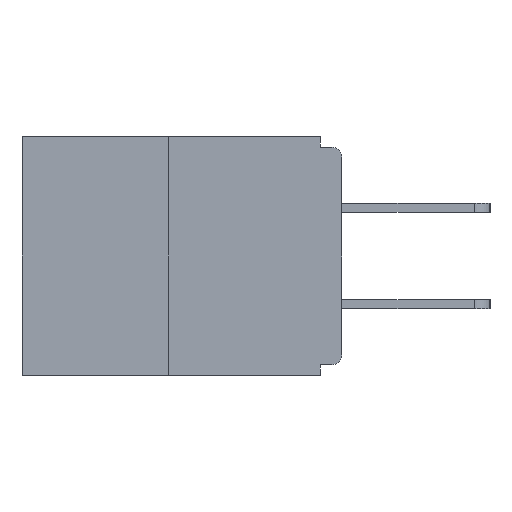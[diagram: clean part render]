
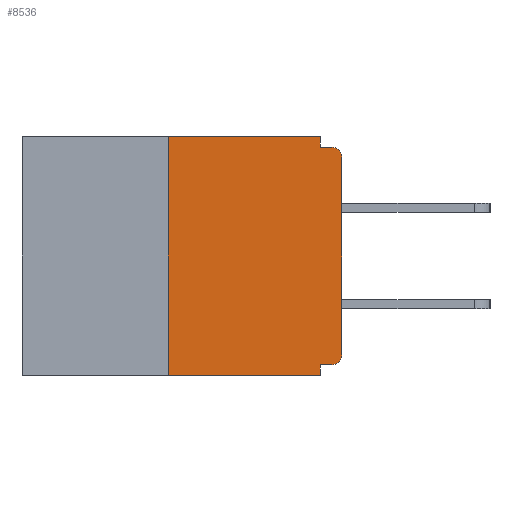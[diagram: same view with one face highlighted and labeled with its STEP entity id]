
A CAD part, left-side view. The second image highlights one B-rep face of the part: STEP entity #8536.
In plain terms, the highlighted planar face has unit normal (-1, 0, 0).
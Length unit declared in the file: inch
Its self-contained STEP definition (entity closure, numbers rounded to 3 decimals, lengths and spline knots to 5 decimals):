
#121 = DIRECTION ( 'NONE',  ( -1., 0., 0. ) ) ;
#288 = DIRECTION ( 'NONE',  ( 0., -1., 0. ) ) ;
#297 = VERTEX_POINT ( 'NONE', #10565 ) ;
#346 = FACE_OUTER_BOUND ( 'NONE', #8840, .T. ) ;
#440 = LINE ( 'NONE', #13650, #11971 ) ;
#607 = DIRECTION ( 'NONE',  ( 0., 0., 1. ) ) ;
#777 = CARTESIAN_POINT ( 'NONE',  ( 0., 0.015, -0.313 ) ) ;
#892 = AXIS2_PLACEMENT_3D ( 'NONE', #9704, #121, #13093 ) ;
#996 = ORIENTED_EDGE ( 'NONE', *, *, #9010, .F. ) ;
#1047 = VERTEX_POINT ( 'NONE', #8521 ) ;
#1098 = CARTESIAN_POINT ( 'NONE',  ( 0., 0.015, -0.328 ) ) ;
#1239 = ORIENTED_EDGE ( 'NONE', *, *, #13432, .F. ) ;
#1295 = ORIENTED_EDGE ( 'NONE', *, *, #5062, .F. ) ;
#1489 = PLANE ( 'NONE',  #9682 ) ;
#1593 = VERTEX_POINT ( 'NONE', #3477 ) ;
#2146 = CARTESIAN_POINT ( 'NONE',  ( 0., 0.25, 0. ) ) ;
#2199 = CARTESIAN_POINT ( 'NONE',  ( 0., 0., -0.03 ) ) ;
#2522 = DIRECTION ( 'NONE',  ( 0., -1., 0. ) ) ;
#2578 = CARTESIAN_POINT ( 'NONE',  ( 0., 0.46, 0. ) ) ;
#2584 = ORIENTED_EDGE ( 'NONE', *, *, #3520, .T. ) ;
#2741 = DIRECTION ( 'NONE',  ( 0., 0., -1. ) ) ;
#3351 = VERTEX_POINT ( 'NONE', #14067 ) ;
#3357 = VERTEX_POINT ( 'NONE', #12933 ) ;
#3477 = CARTESIAN_POINT ( 'NONE',  ( 0., 0.031, -0.343 ) ) ;
#3520 = EDGE_CURVE ( 'NONE', #12485, #3357, #7251, .T. ) ;
#3584 = CARTESIAN_POINT ( 'NONE',  ( 0., 0.46, 0. ) ) ;
#3701 = ORIENTED_EDGE ( 'NONE', *, *, #10935, .F. ) ;
#3854 = DIRECTION ( 'NONE',  ( 0., -1., 0. ) ) ;
#3901 = LINE ( 'NONE', #6438, #13106 ) ;
#4170 = EDGE_CURVE ( 'NONE', #7178, #3351, #13710, .T. ) ;
#4305 = CARTESIAN_POINT ( 'NONE',  ( 0., 0.25, 0. ) ) ;
#4355 = ORIENTED_EDGE ( 'NONE', *, *, #8280, .T. ) ;
#5062 = EDGE_CURVE ( 'NONE', #297, #10849, #440, .T. ) ;
#5086 = DIRECTION ( 'NONE',  ( 0., 0., -1. ) ) ;
#5302 = CARTESIAN_POINT ( 'NONE',  ( 0., 0.031, -0.343 ) ) ;
#5489 = ORIENTED_EDGE ( 'NONE', *, *, #10494, .F. ) ;
#5531 = VECTOR ( 'NONE', #607, 39.37008 ) ;
#5757 = LINE ( 'NONE', #8891, #9996 ) ;
#5879 = CARTESIAN_POINT ( 'NONE',  ( 0., 0.031, -0.328 ) ) ;
#6438 = CARTESIAN_POINT ( 'NONE',  ( 0., 0., 0. ) ) ;
#6779 = VECTOR ( 'NONE', #3854, 39.37008 ) ;
#6799 = DIRECTION ( 'NONE',  ( 0., 1., 0. ) ) ;
#6903 = LINE ( 'NONE', #2146, #5531 ) ;
#7178 = VERTEX_POINT ( 'NONE', #2199 ) ;
#7251 = CIRCLE ( 'NONE', #10456, 0.015 ) ;
#7663 = VECTOR ( 'NONE', #2522, 39.37008 ) ;
#7943 = LINE ( 'NONE', #3584, #13074 ) ;
#8221 = ORIENTED_EDGE ( 'NONE', *, *, #8474, .F. ) ;
#8280 = EDGE_CURVE ( 'NONE', #1047, #1593, #13930, .T. ) ;
#8474 = EDGE_CURVE ( 'NONE', #12485, #11956, #5757, .T. ) ;
#8519 = CARTESIAN_POINT ( 'NONE',  ( 0., 0.031, -0.015 ) ) ;
#8521 = CARTESIAN_POINT ( 'NONE',  ( 0., 0.25, -0.343 ) ) ;
#8536 = ADVANCED_FACE ( 'NONE', ( #346 ), #1489, .F. ) ;
#8538 = DIRECTION ( 'NONE',  ( 0., 0., 1. ) ) ;
#8840 = EDGE_LOOP ( 'NONE', ( #996, #1239, #4355, #3701, #8221, #2584, #9899, #11699, #5489, #1295 ) ) ;
#8869 = LINE ( 'NONE', #10265, #7663 ) ;
#8891 = CARTESIAN_POINT ( 'NONE',  ( 0., 0., -0.328 ) ) ;
#9010 = EDGE_CURVE ( 'NONE', #11221, #297, #7943, .T. ) ;
#9227 = DIRECTION ( 'NONE',  ( 1., 0., 0. ) ) ;
#9370 = CARTESIAN_POINT ( 'NONE',  ( 0., 0.46, -0.343 ) ) ;
#9514 = VECTOR ( 'NONE', #10847, 39.37008 ) ;
#9682 = AXIS2_PLACEMENT_3D ( 'NONE', #2578, #9227, #11400 ) ;
#9704 = CARTESIAN_POINT ( 'NONE',  ( 0., 0.015, -0.03 ) ) ;
#9899 = ORIENTED_EDGE ( 'NONE', *, *, #11284, .T. ) ;
#9996 = VECTOR ( 'NONE', #6799, 39.37008 ) ;
#10265 = CARTESIAN_POINT ( 'NONE',  ( 0., 0., -0.015 ) ) ;
#10456 = AXIS2_PLACEMENT_3D ( 'NONE', #777, #12897, #5086 ) ;
#10494 = EDGE_CURVE ( 'NONE', #10849, #3351, #8869, .T. ) ;
#10565 = CARTESIAN_POINT ( 'NONE',  ( 0., 0.031, 0. ) ) ;
#10847 = DIRECTION ( 'NONE',  ( 0., 0., -1. ) ) ;
#10849 = VERTEX_POINT ( 'NONE', #8519 ) ;
#10935 = EDGE_CURVE ( 'NONE', #11956, #1593, #13292, .T. ) ;
#11221 = VERTEX_POINT ( 'NONE', #4305 ) ;
#11284 = EDGE_CURVE ( 'NONE', #3357, #7178, #3901, .T. ) ;
#11400 = DIRECTION ( 'NONE',  ( 0., 0., -1. ) ) ;
#11699 = ORIENTED_EDGE ( 'NONE', *, *, #4170, .T. ) ;
#11956 = VERTEX_POINT ( 'NONE', #5879 ) ;
#11971 = VECTOR ( 'NONE', #2741, 39.37008 ) ;
#12485 = VERTEX_POINT ( 'NONE', #1098 ) ;
#12897 = DIRECTION ( 'NONE',  ( -1., 0., 0. ) ) ;
#12933 = CARTESIAN_POINT ( 'NONE',  ( 0., 0., -0.313 ) ) ;
#13074 = VECTOR ( 'NONE', #288, 39.37008 ) ;
#13093 = DIRECTION ( 'NONE',  ( 0., 0., -1. ) ) ;
#13106 = VECTOR ( 'NONE', #8538, 39.37008 ) ;
#13292 = LINE ( 'NONE', #5302, #9514 ) ;
#13432 = EDGE_CURVE ( 'NONE', #1047, #11221, #6903, .T. ) ;
#13650 = CARTESIAN_POINT ( 'NONE',  ( 0., 0.031, 0. ) ) ;
#13710 = CIRCLE ( 'NONE', #892, 0.015 ) ;
#13930 = LINE ( 'NONE', #9370, #6779 ) ;
#14067 = CARTESIAN_POINT ( 'NONE',  ( 0., 0.015, -0.015 ) ) ;
